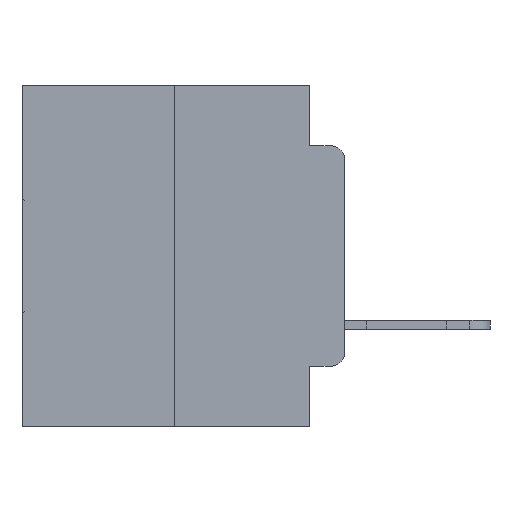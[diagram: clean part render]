
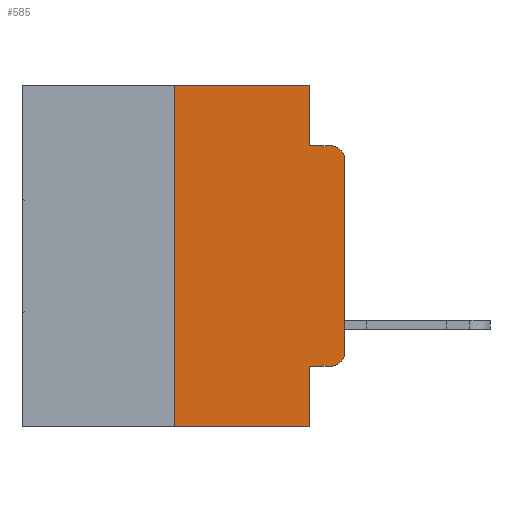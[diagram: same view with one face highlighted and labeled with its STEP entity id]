
A CAD part, left-side view. The second image highlights one B-rep face of the part: STEP entity #585.
In plain terms, the highlighted planar face has unit normal (-1, 0, 0).
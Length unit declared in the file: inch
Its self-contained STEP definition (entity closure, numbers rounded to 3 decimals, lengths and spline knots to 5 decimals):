
#189 = VECTOR ( 'NONE', #11463, 39.37008 ) ;
#585 = ADVANCED_FACE ( 'NONE', ( #14207 ), #6909, .F. ) ;
#818 = EDGE_CURVE ( 'NONE', #16557, #3764, #19178, .T. ) ;
#1398 = CIRCLE ( 'NONE', #6759, 0.02 ) ;
#1838 = DIRECTION ( 'NONE',  ( 1., 0., 0. ) ) ;
#2613 = ORIENTED_EDGE ( 'NONE', *, *, #23578, .T. ) ;
#2694 = VERTEX_POINT ( 'NONE', #8208 ) ;
#2732 = DIRECTION ( 'NONE',  ( 0., 0., -1. ) ) ;
#2782 = CARTESIAN_POINT ( 'NONE',  ( 0., 0.051, -0.4115 ) ) ;
#2800 = CARTESIAN_POINT ( 'NONE',  ( 0., 0.051, 0. ) ) ;
#3231 = DIRECTION ( 'NONE',  ( 0., 0., -1. ) ) ;
#3364 = CARTESIAN_POINT ( 'NONE',  ( 0., 0.051, 0. ) ) ;
#3417 = AXIS2_PLACEMENT_3D ( 'NONE', #4704, #1838, #5723 ) ;
#3635 = EDGE_CURVE ( 'NONE', #18938, #4728, #8211, .T. ) ;
#3755 = DIRECTION ( 'NONE',  ( 0., -1., 0. ) ) ;
#3764 = VERTEX_POINT ( 'NONE', #5699 ) ;
#4704 = CARTESIAN_POINT ( 'NONE',  ( 0., 0.473, 0. ) ) ;
#4728 = VERTEX_POINT ( 'NONE', #12446 ) ;
#5699 = CARTESIAN_POINT ( 'NONE',  ( 0., 0.051, -0.5 ) ) ;
#5723 = DIRECTION ( 'NONE',  ( 0., 0., -1. ) ) ;
#6612 = ORIENTED_EDGE ( 'NONE', *, *, #3635, .T. ) ;
#6759 = AXIS2_PLACEMENT_3D ( 'NONE', #8387, #8360, #8326 ) ;
#6909 = PLANE ( 'NONE',  #3417 ) ;
#7116 = CARTESIAN_POINT ( 'NONE',  ( 0., 0.25, -0.5 ) ) ;
#7131 = LINE ( 'NONE', #11359, #189 ) ;
#7455 = DIRECTION ( 'NONE',  ( 0., -1., 0. ) ) ;
#7487 = VERTEX_POINT ( 'NONE', #26358 ) ;
#7600 = CARTESIAN_POINT ( 'NONE',  ( 0., 0.051, -0.0885 ) ) ;
#7811 = LINE ( 'NONE', #23948, #23480 ) ;
#8158 = VERTEX_POINT ( 'NONE', #8990 ) ;
#8208 = CARTESIAN_POINT ( 'NONE',  ( 0., 0., -0.1085 ) ) ;
#8211 = CIRCLE ( 'NONE', #10589, 0.02 ) ;
#8275 = VECTOR ( 'NONE', #23585, 39.37008 ) ;
#8326 = DIRECTION ( 'NONE',  ( 0., 0., -1. ) ) ;
#8360 = DIRECTION ( 'NONE',  ( -1., 0., 0. ) ) ;
#8387 = CARTESIAN_POINT ( 'NONE',  ( 0., 0.02, -0.1085 ) ) ;
#8559 = DIRECTION ( 'NONE',  ( -1., 0., 0. ) ) ;
#8990 = CARTESIAN_POINT ( 'NONE',  ( 0., 0.25, 0. ) ) ;
#9443 = CARTESIAN_POINT ( 'NONE',  ( 0., 0.051, 0. ) ) ;
#10058 = VECTOR ( 'NONE', #14812, 39.37008 ) ;
#10416 = CARTESIAN_POINT ( 'NONE',  ( 0., 0.02, -0.0885 ) ) ;
#10589 = AXIS2_PLACEMENT_3D ( 'NONE', #12781, #8559, #3231 ) ;
#10940 = ORIENTED_EDGE ( 'NONE', *, *, #818, .T. ) ;
#11309 = VERTEX_POINT ( 'NONE', #10416 ) ;
#11359 = CARTESIAN_POINT ( 'NONE',  ( 0., 0., 0. ) ) ;
#11463 = DIRECTION ( 'NONE',  ( 0., 0., 1. ) ) ;
#12302 = EDGE_LOOP ( 'NONE', ( #29395, #2613, #21451, #13395, #19199, #22288, #10940, #16124, #20345, #6612 ) ) ;
#12342 = VECTOR ( 'NONE', #3755, 39.37008 ) ;
#12446 = CARTESIAN_POINT ( 'NONE',  ( 0., 0., -0.3915 ) ) ;
#12481 = CARTESIAN_POINT ( 'NONE',  ( 0., 0.473, 0. ) ) ;
#12609 = VECTOR ( 'NONE', #7455, 39.37008 ) ;
#12781 = CARTESIAN_POINT ( 'NONE',  ( 0., 0.02, -0.3915 ) ) ;
#13387 = LINE ( 'NONE', #7600, #12609 ) ;
#13395 = ORIENTED_EDGE ( 'NONE', *, *, #23842, .F. ) ;
#14207 = FACE_OUTER_BOUND ( 'NONE', #12302, .T. ) ;
#14812 = DIRECTION ( 'NONE',  ( 0., -1., 0. ) ) ;
#16124 = ORIENTED_EDGE ( 'NONE', *, *, #24600, .F. ) ;
#16557 = VERTEX_POINT ( 'NONE', #7116 ) ;
#17647 = VERTEX_POINT ( 'NONE', #9443 ) ;
#18938 = VERTEX_POINT ( 'NONE', #18952 ) ;
#18952 = CARTESIAN_POINT ( 'NONE',  ( 0., 0.02, -0.4115 ) ) ;
#19178 = LINE ( 'NONE', #26415, #12342 ) ;
#19199 = ORIENTED_EDGE ( 'NONE', *, *, #29957, .F. ) ;
#20345 = ORIENTED_EDGE ( 'NONE', *, *, #25041, .T. ) ;
#20715 = LINE ( 'NONE', #30108, #8275 ) ;
#21451 = ORIENTED_EDGE ( 'NONE', *, *, #23613, .F. ) ;
#22269 = LINE ( 'NONE', #12481, #10058 ) ;
#22288 = ORIENTED_EDGE ( 'NONE', *, *, #24321, .F. ) ;
#22456 = DIRECTION ( 'NONE',  ( 0., 0., -1. ) ) ;
#22826 = VECTOR ( 'NONE', #2732, 39.37008 ) ;
#23440 = EDGE_CURVE ( 'NONE', #4728, #2694, #7131, .T. ) ;
#23480 = VECTOR ( 'NONE', #26206, 39.37008 ) ;
#23578 = EDGE_CURVE ( 'NONE', #2694, #11309, #1398, .T. ) ;
#23585 = DIRECTION ( 'NONE',  ( 0., 0., 1. ) ) ;
#23613 = EDGE_CURVE ( 'NONE', #7487, #11309, #13387, .T. ) ;
#23842 = EDGE_CURVE ( 'NONE', #17647, #7487, #28759, .T. ) ;
#23948 = CARTESIAN_POINT ( 'NONE',  ( 0., 0.051, -0.4115 ) ) ;
#24234 = LINE ( 'NONE', #3364, #29962 ) ;
#24321 = EDGE_CURVE ( 'NONE', #16557, #8158, #20715, .T. ) ;
#24497 = VERTEX_POINT ( 'NONE', #2782 ) ;
#24600 = EDGE_CURVE ( 'NONE', #24497, #3764, #24234, .T. ) ;
#25041 = EDGE_CURVE ( 'NONE', #24497, #18938, #7811, .T. ) ;
#26206 = DIRECTION ( 'NONE',  ( 0., -1., 0. ) ) ;
#26358 = CARTESIAN_POINT ( 'NONE',  ( 0., 0.051, -0.0885 ) ) ;
#26415 = CARTESIAN_POINT ( 'NONE',  ( 0., 0.473, -0.5 ) ) ;
#28759 = LINE ( 'NONE', #2800, #22826 ) ;
#29395 = ORIENTED_EDGE ( 'NONE', *, *, #23440, .T. ) ;
#29957 = EDGE_CURVE ( 'NONE', #8158, #17647, #22269, .T. ) ;
#29962 = VECTOR ( 'NONE', #22456, 39.37008 ) ;
#30108 = CARTESIAN_POINT ( 'NONE',  ( 0., 0.25, 0. ) ) ;
